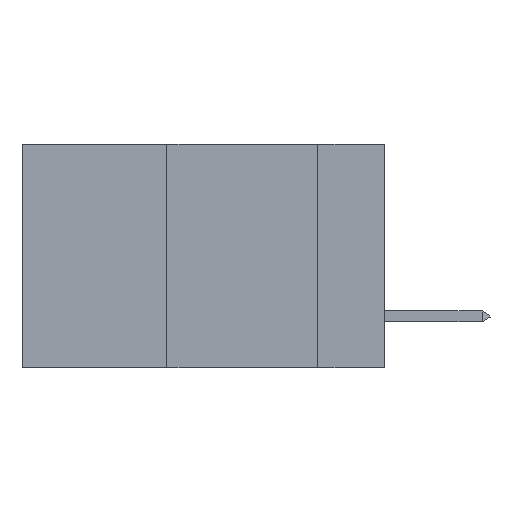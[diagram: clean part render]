
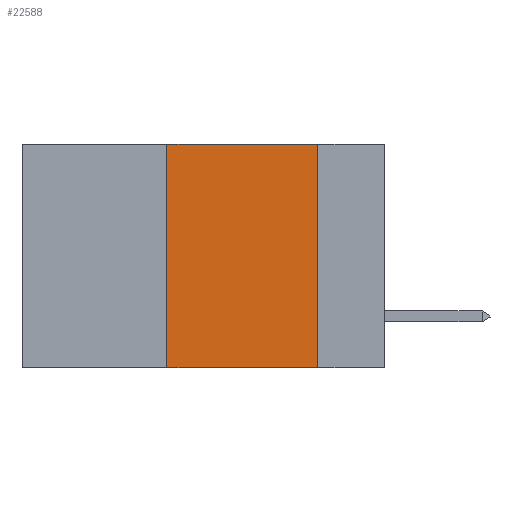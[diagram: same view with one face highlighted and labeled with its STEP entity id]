
A CAD part, left-side view. The second image highlights one B-rep face of the part: STEP entity #22588.
In plain terms, the highlighted planar face has unit normal (-1, 0, 0).
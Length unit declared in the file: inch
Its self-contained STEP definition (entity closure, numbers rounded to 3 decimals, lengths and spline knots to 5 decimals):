
#2717 = CARTESIAN_POINT ( 'NONE',  ( 0., 0.11, 0. ) ) ;
#7349 = LINE ( 'NONE', #19202, #10177 ) ;
#7766 = DIRECTION ( 'NONE',  ( 1., 0., 0. ) ) ;
#7929 = CARTESIAN_POINT ( 'NONE',  ( 0., 0.6, 0. ) ) ;
#9695 = EDGE_CURVE ( 'NONE', #22121, #36541, #37691, .T. ) ;
#10177 = VECTOR ( 'NONE', #22860, 39.37008 ) ;
#11699 = LINE ( 'NONE', #38966, #17925 ) ;
#13469 = CARTESIAN_POINT ( 'NONE',  ( 0., 0.11, -0.37 ) ) ;
#14797 = CARTESIAN_POINT ( 'NONE',  ( 0., 0.11, 0. ) ) ;
#15440 = VECTOR ( 'NONE', #28269, 39.37008 ) ;
#16295 = VECTOR ( 'NONE', #22287, 39.37008 ) ;
#16983 = EDGE_CURVE ( 'NONE', #41978, #36541, #7349, .T. ) ;
#17082 = DIRECTION ( 'NONE',  ( 0., 0., 1. ) ) ;
#17925 = VECTOR ( 'NONE', #17082, 39.37008 ) ;
#19202 = CARTESIAN_POINT ( 'NONE',  ( 0., 0.6, -0.37 ) ) ;
#21346 = CARTESIAN_POINT ( 'NONE',  ( 0., 0.36, 0. ) ) ;
#21485 = AXIS2_PLACEMENT_3D ( 'NONE', #7929, #7766, #40022 ) ;
#22121 = VERTEX_POINT ( 'NONE', #14797 ) ;
#22287 = DIRECTION ( 'NONE',  ( 0., -1., 0. ) ) ;
#22492 = ORIENTED_EDGE ( 'NONE', *, *, #42790, .F. ) ;
#22588 = ADVANCED_FACE ( 'NONE', ( #27349 ), #33021, .F. ) ;
#22860 = DIRECTION ( 'NONE',  ( 0., -1., 0. ) ) ;
#24385 = VERTEX_POINT ( 'NONE', #21346 ) ;
#27349 = FACE_OUTER_BOUND ( 'NONE', #38932, .T. ) ;
#27973 = EDGE_CURVE ( 'NONE', #24385, #22121, #41999, .T. ) ;
#28269 = DIRECTION ( 'NONE',  ( 0., 0., -1. ) ) ;
#30262 = CARTESIAN_POINT ( 'NONE',  ( 0., 0.36, -0.37 ) ) ;
#33021 = PLANE ( 'NONE',  #21485 ) ;
#36152 = CARTESIAN_POINT ( 'NONE',  ( 0., 0.6, 0. ) ) ;
#36541 = VERTEX_POINT ( 'NONE', #13469 ) ;
#37272 = ORIENTED_EDGE ( 'NONE', *, *, #9695, .F. ) ;
#37691 = LINE ( 'NONE', #2717, #15440 ) ;
#38932 = EDGE_LOOP ( 'NONE', ( #37272, #45195, #22492, #41426 ) ) ;
#38966 = CARTESIAN_POINT ( 'NONE',  ( 0., 0.36, 0. ) ) ;
#40022 = DIRECTION ( 'NONE',  ( 0., 0., -1. ) ) ;
#41426 = ORIENTED_EDGE ( 'NONE', *, *, #16983, .T. ) ;
#41978 = VERTEX_POINT ( 'NONE', #30262 ) ;
#41999 = LINE ( 'NONE', #36152, #16295 ) ;
#42790 = EDGE_CURVE ( 'NONE', #41978, #24385, #11699, .T. ) ;
#45195 = ORIENTED_EDGE ( 'NONE', *, *, #27973, .F. ) ;
